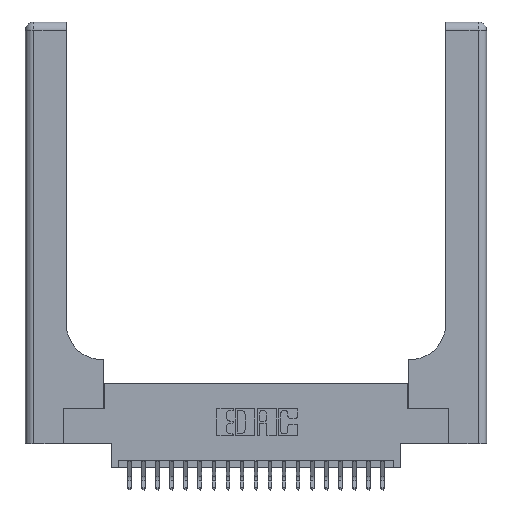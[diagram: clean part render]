
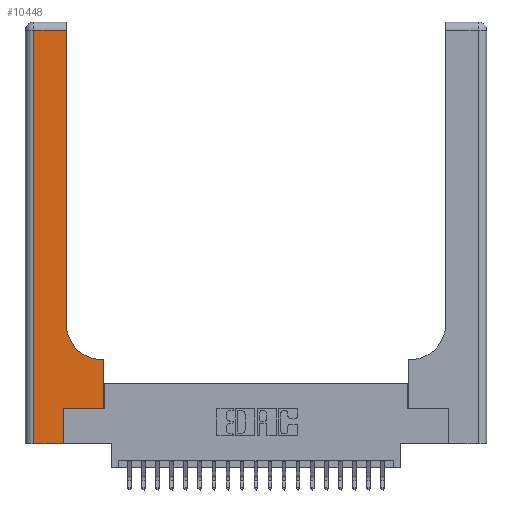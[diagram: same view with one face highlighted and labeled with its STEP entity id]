
A CAD part, top view. The second image highlights one B-rep face of the part: STEP entity #10448.
In plain terms, the highlighted planar face has unit normal (0, 0, 1).
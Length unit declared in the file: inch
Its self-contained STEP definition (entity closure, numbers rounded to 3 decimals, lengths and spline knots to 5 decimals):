
#17 = VECTOR ( 'NONE', #18140, 39.37008 ) ;
#127 = CARTESIAN_POINT ( 'NONE',  ( 0., 2.94, 0.37 ) ) ;
#270 = EDGE_CURVE ( 'NONE', #23034, #22955, #1875, .T. ) ;
#290 = CARTESIAN_POINT ( 'NONE',  ( 0.269, 0.25, 0.37 ) ) ;
#709 = VECTOR ( 'NONE', #4459, 39.37008 ) ;
#716 = DIRECTION ( 'NONE',  ( 0., 0., -1. ) ) ;
#1060 = CARTESIAN_POINT ( 'NONE',  ( 0.06, 2.94, 0.37 ) ) ;
#1085 = VECTOR ( 'NONE', #16058, 39.37008 ) ;
#1409 = LINE ( 'NONE', #23482, #20775 ) ;
#1875 = LINE ( 'NONE', #4650, #709 ) ;
#3356 = CARTESIAN_POINT ( 'NONE',  ( 0.2915, 3., 0.37 ) ) ;
#3384 = ORIENTED_EDGE ( 'NONE', *, *, #20511, .T. ) ;
#3481 = CARTESIAN_POINT ( 'NONE',  ( 0., 3., 0.37 ) ) ;
#3560 = DIRECTION ( 'NONE',  ( 0., 1., 0. ) ) ;
#4459 = DIRECTION ( 'NONE',  ( 0., 1., 0. ) ) ;
#4583 = LINE ( 'NONE', #10977, #13672 ) ;
#4604 = CIRCLE ( 'NONE', #19459, 0.25 ) ;
#4650 = CARTESIAN_POINT ( 'NONE',  ( 0.5585, 0.25, 0.37 ) ) ;
#4807 = CARTESIAN_POINT ( 'NONE',  ( 0.5585, 0.6, 0.37 ) ) ;
#4894 = EDGE_CURVE ( 'NONE', #17571, #18881, #1409, .T. ) ;
#5544 = DIRECTION ( 'NONE',  ( 0., -1., 0. ) ) ;
#5733 = ORIENTED_EDGE ( 'NONE', *, *, #270, .T. ) ;
#6093 = FACE_OUTER_BOUND ( 'NONE', #14938, .T. ) ;
#7215 = PLANE ( 'NONE',  #14801 ) ;
#7241 = CARTESIAN_POINT ( 'NONE',  ( 0.06, 3., 0.37 ) ) ;
#7744 = ORIENTED_EDGE ( 'NONE', *, *, #22500, .T. ) ;
#7828 = VECTOR ( 'NONE', #11166, 39.37008 ) ;
#8302 = VERTEX_POINT ( 'NONE', #21061 ) ;
#8393 = LINE ( 'NONE', #127, #7828 ) ;
#9143 = CARTESIAN_POINT ( 'NONE',  ( 0., 0., 0.37 ) ) ;
#9429 = ORIENTED_EDGE ( 'NONE', *, *, #4894, .T. ) ;
#10324 = LINE ( 'NONE', #3356, #1085 ) ;
#10448 = ADVANCED_FACE ( 'NONE', ( #6093 ), #7215, .F. ) ;
#10566 = CARTESIAN_POINT ( 'NONE',  ( 0.269, 0.25, 0.37 ) ) ;
#10848 = DIRECTION ( 'NONE',  ( 0., 0., -1. ) ) ;
#10951 = CARTESIAN_POINT ( 'NONE',  ( 0.2915, 0.85, 0.37 ) ) ;
#10977 = CARTESIAN_POINT ( 'NONE',  ( 0.2915, 0.6, 0.37 ) ) ;
#11166 = DIRECTION ( 'NONE',  ( -1., 0., 0. ) ) ;
#11421 = VERTEX_POINT ( 'NONE', #19819 ) ;
#11447 = VERTEX_POINT ( 'NONE', #10951 ) ;
#11454 = EDGE_CURVE ( 'NONE', #17951, #21710, #18750, .T. ) ;
#11694 = ORIENTED_EDGE ( 'NONE', *, *, #22861, .T. ) ;
#11744 = CARTESIAN_POINT ( 'NONE',  ( 0.5415, 0.85, 0.37 ) ) ;
#12202 = CARTESIAN_POINT ( 'NONE',  ( 0.5585, 0.25, 0.37 ) ) ;
#12393 = DIRECTION ( 'NONE',  ( 1., 0., 0. ) ) ;
#12794 = DIRECTION ( 'NONE',  ( -1., 0., 0. ) ) ;
#13559 = DIRECTION ( 'NONE',  ( 1., 0., 0. ) ) ;
#13672 = VECTOR ( 'NONE', #12794, 39.37008 ) ;
#14327 = VECTOR ( 'NONE', #12393, 39.37008 ) ;
#14597 = LINE ( 'NONE', #10566, #14327 ) ;
#14767 = ORIENTED_EDGE ( 'NONE', *, *, #21612, .T. ) ;
#14801 = AXIS2_PLACEMENT_3D ( 'NONE', #3481, #10848, #23396 ) ;
#14890 = EDGE_CURVE ( 'NONE', #22955, #11421, #4583, .T. ) ;
#14938 = EDGE_LOOP ( 'NONE', ( #7744, #3384, #22641, #18444, #9429, #14767, #5733, #20687, #11694 ) ) ;
#16058 = DIRECTION ( 'NONE',  ( 0., 1., 0. ) ) ;
#17571 = VERTEX_POINT ( 'NONE', #18086 ) ;
#17951 = VERTEX_POINT ( 'NONE', #1060 ) ;
#18048 = CARTESIAN_POINT ( 'NONE',  ( 0.06, 0., 0.37 ) ) ;
#18086 = CARTESIAN_POINT ( 'NONE',  ( 0.269, 0., 0.37 ) ) ;
#18102 = EDGE_CURVE ( 'NONE', #21710, #17571, #19998, .T. ) ;
#18140 = DIRECTION ( 'NONE',  ( 1., 0., 0. ) ) ;
#18189 = VECTOR ( 'NONE', #5544, 39.37008 ) ;
#18444 = ORIENTED_EDGE ( 'NONE', *, *, #18102, .T. ) ;
#18750 = LINE ( 'NONE', #7241, #18189 ) ;
#18881 = VERTEX_POINT ( 'NONE', #290 ) ;
#19459 = AXIS2_PLACEMENT_3D ( 'NONE', #11744, #716, #13559 ) ;
#19819 = CARTESIAN_POINT ( 'NONE',  ( 0.5415, 0.6, 0.37 ) ) ;
#19998 = LINE ( 'NONE', #9143, #17 ) ;
#20511 = EDGE_CURVE ( 'NONE', #8302, #17951, #8393, .T. ) ;
#20687 = ORIENTED_EDGE ( 'NONE', *, *, #14890, .T. ) ;
#20775 = VECTOR ( 'NONE', #3560, 39.37008 ) ;
#21061 = CARTESIAN_POINT ( 'NONE',  ( 0.2915, 2.94, 0.37 ) ) ;
#21612 = EDGE_CURVE ( 'NONE', #18881, #23034, #14597, .T. ) ;
#21710 = VERTEX_POINT ( 'NONE', #18048 ) ;
#22500 = EDGE_CURVE ( 'NONE', #11447, #8302, #10324, .T. ) ;
#22641 = ORIENTED_EDGE ( 'NONE', *, *, #11454, .T. ) ;
#22861 = EDGE_CURVE ( 'NONE', #11421, #11447, #4604, .T. ) ;
#22955 = VERTEX_POINT ( 'NONE', #4807 ) ;
#23034 = VERTEX_POINT ( 'NONE', #12202 ) ;
#23396 = DIRECTION ( 'NONE',  ( -1., 0., 0. ) ) ;
#23482 = CARTESIAN_POINT ( 'NONE',  ( 0.269, 0., 0.37 ) ) ;
